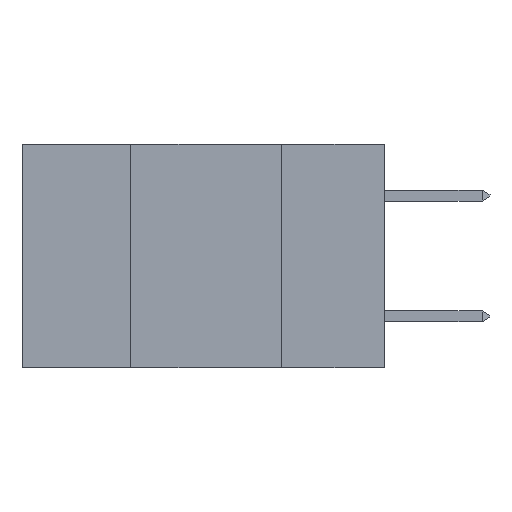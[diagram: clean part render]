
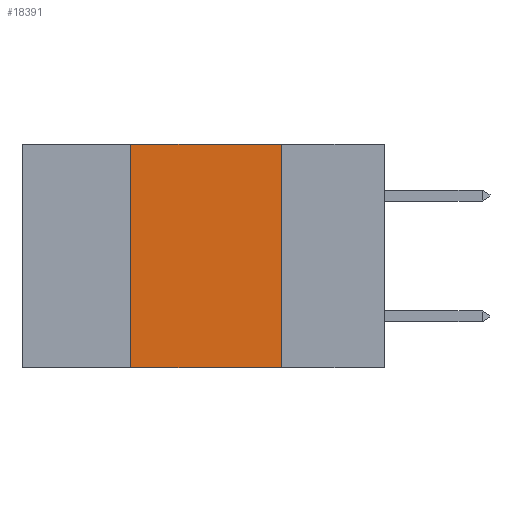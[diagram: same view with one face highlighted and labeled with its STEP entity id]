
A CAD part, left-side view. The second image highlights one B-rep face of the part: STEP entity #18391.
In plain terms, the highlighted planar face has unit normal (-1, 0, 0).
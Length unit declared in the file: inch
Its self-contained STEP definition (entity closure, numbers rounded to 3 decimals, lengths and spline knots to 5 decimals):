
#326 = DIRECTION ( 'NONE',  ( 0., -1., 0. ) ) ;
#1107 = DIRECTION ( 'NONE',  ( 1., 0., 0. ) ) ;
#1240 = EDGE_CURVE ( 'NONE', #23318, #12529, #2368, .T. ) ;
#1474 = DIRECTION ( 'NONE',  ( 0., 0., -1. ) ) ;
#2290 = LINE ( 'NONE', #2407, #21940 ) ;
#2368 = LINE ( 'NONE', #18691, #3002 ) ;
#2407 = CARTESIAN_POINT ( 'NONE',  ( 0., 0.6, -0.37 ) ) ;
#2565 = EDGE_CURVE ( 'NONE', #15374, #18617, #2290, .T. ) ;
#2650 = FACE_OUTER_BOUND ( 'NONE', #9918, .T. ) ;
#3002 = VECTOR ( 'NONE', #24804, 39.37008 ) ;
#3153 = DIRECTION ( 'NONE',  ( 0., 0., -1. ) ) ;
#4092 = CARTESIAN_POINT ( 'NONE',  ( 0., 0.42, -0.37 ) ) ;
#4293 = VECTOR ( 'NONE', #23842, 39.37008 ) ;
#4392 = AXIS2_PLACEMENT_3D ( 'NONE', #7458, #1107, #3153 ) ;
#5365 = EDGE_CURVE ( 'NONE', #12529, #18617, #10386, .T. ) ;
#7458 = CARTESIAN_POINT ( 'NONE',  ( 0., 0.6, 0. ) ) ;
#9918 = EDGE_LOOP ( 'NONE', ( #18832, #24158, #18169, #24439 ) ) ;
#10386 = LINE ( 'NONE', #26045, #14288 ) ;
#10506 = CARTESIAN_POINT ( 'NONE',  ( 0., 0.17, 0. ) ) ;
#12529 = VERTEX_POINT ( 'NONE', #10506 ) ;
#14288 = VECTOR ( 'NONE', #1474, 39.37008 ) ;
#15374 = VERTEX_POINT ( 'NONE', #4092 ) ;
#16301 = CARTESIAN_POINT ( 'NONE',  ( 0., 0.17, -0.37 ) ) ;
#18169 = ORIENTED_EDGE ( 'NONE', *, *, #22513, .F. ) ;
#18391 = ADVANCED_FACE ( 'NONE', ( #2650 ), #19547, .F. ) ;
#18617 = VERTEX_POINT ( 'NONE', #16301 ) ;
#18691 = CARTESIAN_POINT ( 'NONE',  ( 0., 0.6, 0. ) ) ;
#18832 = ORIENTED_EDGE ( 'NONE', *, *, #5365, .F. ) ;
#19547 = PLANE ( 'NONE',  #4392 ) ;
#20605 = CARTESIAN_POINT ( 'NONE',  ( 0., 0.42, 0. ) ) ;
#21832 = CARTESIAN_POINT ( 'NONE',  ( 0., 0.42, 0. ) ) ;
#21940 = VECTOR ( 'NONE', #326, 39.37008 ) ;
#22513 = EDGE_CURVE ( 'NONE', #15374, #23318, #25183, .T. ) ;
#23318 = VERTEX_POINT ( 'NONE', #20605 ) ;
#23842 = DIRECTION ( 'NONE',  ( 0., 0., 1. ) ) ;
#24158 = ORIENTED_EDGE ( 'NONE', *, *, #1240, .F. ) ;
#24439 = ORIENTED_EDGE ( 'NONE', *, *, #2565, .T. ) ;
#24804 = DIRECTION ( 'NONE',  ( 0., -1., 0. ) ) ;
#25183 = LINE ( 'NONE', #21832, #4293 ) ;
#26045 = CARTESIAN_POINT ( 'NONE',  ( 0., 0.17, 0. ) ) ;
